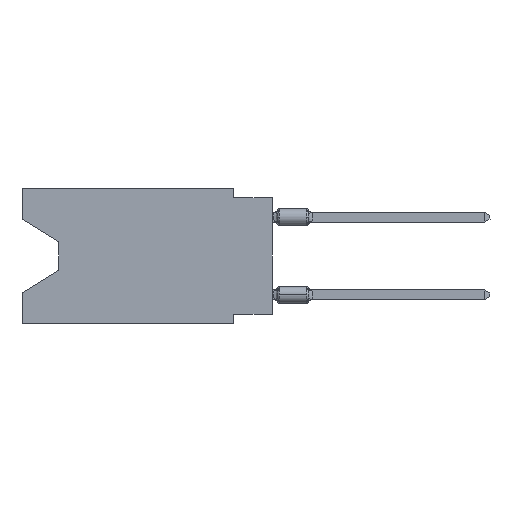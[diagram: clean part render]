
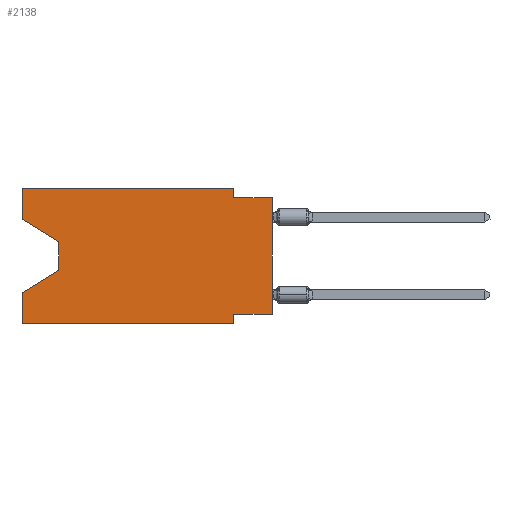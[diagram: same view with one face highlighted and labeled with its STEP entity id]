
A CAD part, left-side view. The second image highlights one B-rep face of the part: STEP entity #2138.
In plain terms, the highlighted planar face has unit normal (-1, 0, 0).
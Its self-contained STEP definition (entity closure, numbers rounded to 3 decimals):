
#279 = EDGE_CURVE ( 'NONE', #19976, #6703, #7703, .T. ) ;
#341 = VECTOR ( 'NONE', #6733, 1000. ) ;
#351 = EDGE_CURVE ( 'NONE', #24159, #17937, #6500, .T. ) ;
#398 = EDGE_CURVE ( 'NONE', #13247, #6703, #24025, .T. ) ;
#952 = VECTOR ( 'NONE', #2241, 1000. ) ;
#1047 = VERTEX_POINT ( 'NONE', #21599 ) ;
#1485 = LINE ( 'NONE', #13294, #25168 ) ;
#1803 = VECTOR ( 'NONE', #21344, 1000. ) ;
#2012 = ORIENTED_EDGE ( 'NONE', *, *, #24083, .T. ) ;
#2138 = ADVANCED_FACE ( 'NONE', ( #20572 ), #8551, .F. ) ;
#2241 = DIRECTION ( 'NONE',  ( 0., 0., -1. ) ) ;
#2556 = CARTESIAN_POINT ( 'NONE',  ( 0., 16.383, 0. ) ) ;
#3279 = DIRECTION ( 'NONE',  ( 0., -1., 0. ) ) ;
#3994 = VECTOR ( 'NONE', #8609, 1000. ) ;
#4396 = VERTEX_POINT ( 'NONE', #18026 ) ;
#4489 = DIRECTION ( 'NONE',  ( 0., 0., -1. ) ) ;
#4534 = CARTESIAN_POINT ( 'NONE',  ( 0., 13.97, -5.385 ) ) ;
#4688 = VERTEX_POINT ( 'NONE', #23330 ) ;
#5049 = EDGE_CURVE ( 'NONE', #1047, #4688, #25258, .T. ) ;
#5396 = CARTESIAN_POINT ( 'NONE',  ( 0., 0., -8.255 ) ) ;
#5401 = VECTOR ( 'NONE', #22063, 1000. ) ;
#5454 = DIRECTION ( 'NONE',  ( 0., -1., 0. ) ) ;
#5958 = CARTESIAN_POINT ( 'NONE',  ( 0., 2.54, 0. ) ) ;
#6413 = CARTESIAN_POINT ( 'NONE',  ( 0., 13.97, -5.385 ) ) ;
#6471 = CARTESIAN_POINT ( 'NONE',  ( 0., 16.383, -6.852 ) ) ;
#6500 = LINE ( 'NONE', #4534, #7056 ) ;
#6703 = VERTEX_POINT ( 'NONE', #14191 ) ;
#6733 = DIRECTION ( 'NONE',  ( 0., 0., -1. ) ) ;
#7056 = VECTOR ( 'NONE', #20498, 1000. ) ;
#7703 = LINE ( 'NONE', #13478, #10817 ) ;
#7768 = ORIENTED_EDGE ( 'NONE', *, *, #398, .T. ) ;
#8443 = CARTESIAN_POINT ( 'NONE',  ( 0., 13.97, -3.505 ) ) ;
#8551 = PLANE ( 'NONE',  #21887 ) ;
#8609 = DIRECTION ( 'NONE',  ( 0., 0., 1. ) ) ;
#8670 = VECTOR ( 'NONE', #3279, 1000. ) ;
#8965 = ORIENTED_EDGE ( 'NONE', *, *, #24908, .T. ) ;
#8996 = ORIENTED_EDGE ( 'NONE', *, *, #23305, .F. ) ;
#9222 = CARTESIAN_POINT ( 'NONE',  ( 0., 0., -8.255 ) ) ;
#10467 = EDGE_CURVE ( 'NONE', #21750, #16307, #1485, .T. ) ;
#10817 = VECTOR ( 'NONE', #15695, 1000. ) ;
#11656 = LINE ( 'NONE', #23662, #12410 ) ;
#12208 = LINE ( 'NONE', #20171, #952 ) ;
#12406 = EDGE_LOOP ( 'NONE', ( #2012, #8965, #16664, #14299, #18149, #13295, #14935, #7768, #24178, #8996, #15888, #23071 ) ) ;
#12410 = VECTOR ( 'NONE', #13745, 1000. ) ;
#13208 = CARTESIAN_POINT ( 'NONE',  ( 0., 13.97, -3.505 ) ) ;
#13247 = VERTEX_POINT ( 'NONE', #9222 ) ;
#13269 = LINE ( 'NONE', #5396, #1803 ) ;
#13294 = CARTESIAN_POINT ( 'NONE',  ( 0., 16.383, 0. ) ) ;
#13295 = ORIENTED_EDGE ( 'NONE', *, *, #18430, .F. ) ;
#13478 = CARTESIAN_POINT ( 'NONE',  ( 0., 0., -0.635 ) ) ;
#13745 = DIRECTION ( 'NONE',  ( 0., 0., -1. ) ) ;
#13830 = CARTESIAN_POINT ( 'NONE',  ( 0., 16.383, 0. ) ) ;
#14090 = VERTEX_POINT ( 'NONE', #5958 ) ;
#14112 = CARTESIAN_POINT ( 'NONE',  ( 0., 0., 0. ) ) ;
#14191 = CARTESIAN_POINT ( 'NONE',  ( 0., 0., -0.635 ) ) ;
#14299 = ORIENTED_EDGE ( 'NONE', *, *, #22031, .F. ) ;
#14364 = LINE ( 'NONE', #2556, #3994 ) ;
#14438 = DIRECTION ( 'NONE',  ( 1., 0., 0. ) ) ;
#14832 = CARTESIAN_POINT ( 'NONE',  ( 0., 16.383, 0. ) ) ;
#14935 = ORIENTED_EDGE ( 'NONE', *, *, #18643, .F. ) ;
#15275 = VERTEX_POINT ( 'NONE', #13208 ) ;
#15591 = CARTESIAN_POINT ( 'NONE',  ( 0., 16.383, -8.89 ) ) ;
#15695 = DIRECTION ( 'NONE',  ( 0., -1., 0. ) ) ;
#15888 = ORIENTED_EDGE ( 'NONE', *, *, #17829, .F. ) ;
#16307 = VERTEX_POINT ( 'NONE', #23262 ) ;
#16664 = ORIENTED_EDGE ( 'NONE', *, *, #351, .T. ) ;
#17829 = EDGE_CURVE ( 'NONE', #16307, #14090, #23492, .T. ) ;
#17937 = VERTEX_POINT ( 'NONE', #6471 ) ;
#18026 = CARTESIAN_POINT ( 'NONE',  ( 0., 2.54, -8.255 ) ) ;
#18149 = ORIENTED_EDGE ( 'NONE', *, *, #5049, .T. ) ;
#18430 = EDGE_CURVE ( 'NONE', #4396, #4688, #12208, .T. ) ;
#18643 = EDGE_CURVE ( 'NONE', #13247, #4396, #13269, .T. ) ;
#18659 = LINE ( 'NONE', #8443, #341 ) ;
#19278 = CARTESIAN_POINT ( 'NONE',  ( 0., 2.54, -0.635 ) ) ;
#19437 = LINE ( 'NONE', #25553, #21661 ) ;
#19976 = VERTEX_POINT ( 'NONE', #19278 ) ;
#20171 = CARTESIAN_POINT ( 'NONE',  ( 0., 2.54, -8.89 ) ) ;
#20498 = DIRECTION ( 'NONE',  ( 0., 0.855, -0.519 ) ) ;
#20572 = FACE_OUTER_BOUND ( 'NONE', #12406, .T. ) ;
#20998 = VECTOR ( 'NONE', #5454, 1000. ) ;
#21344 = DIRECTION ( 'NONE',  ( 0., 1., 0. ) ) ;
#21599 = CARTESIAN_POINT ( 'NONE',  ( 0., 16.383, -8.89 ) ) ;
#21661 = VECTOR ( 'NONE', #23349, 1000. ) ;
#21750 = VERTEX_POINT ( 'NONE', #24313 ) ;
#21887 = AXIS2_PLACEMENT_3D ( 'NONE', #14832, #14438, #4489 ) ;
#22031 = EDGE_CURVE ( 'NONE', #1047, #17937, #14364, .T. ) ;
#22063 = DIRECTION ( 'NONE',  ( 0., 0., 1. ) ) ;
#23071 = ORIENTED_EDGE ( 'NONE', *, *, #10467, .F. ) ;
#23262 = CARTESIAN_POINT ( 'NONE',  ( 0., 16.383, 0. ) ) ;
#23305 = EDGE_CURVE ( 'NONE', #14090, #19976, #11656, .T. ) ;
#23330 = CARTESIAN_POINT ( 'NONE',  ( 0., 2.54, -8.89 ) ) ;
#23337 = DIRECTION ( 'NONE',  ( 0., 0., 1. ) ) ;
#23349 = DIRECTION ( 'NONE',  ( 0., -0.855, -0.519 ) ) ;
#23492 = LINE ( 'NONE', #13830, #20998 ) ;
#23662 = CARTESIAN_POINT ( 'NONE',  ( 0., 2.54, 0. ) ) ;
#24025 = LINE ( 'NONE', #14112, #5401 ) ;
#24083 = EDGE_CURVE ( 'NONE', #21750, #15275, #19437, .T. ) ;
#24159 = VERTEX_POINT ( 'NONE', #6413 ) ;
#24178 = ORIENTED_EDGE ( 'NONE', *, *, #279, .F. ) ;
#24313 = CARTESIAN_POINT ( 'NONE',  ( 0., 16.383, -2.038 ) ) ;
#24908 = EDGE_CURVE ( 'NONE', #15275, #24159, #18659, .T. ) ;
#25168 = VECTOR ( 'NONE', #23337, 1000. ) ;
#25258 = LINE ( 'NONE', #15591, #8670 ) ;
#25553 = CARTESIAN_POINT ( 'NONE',  ( 0., 16.383, -2.038 ) ) ;
